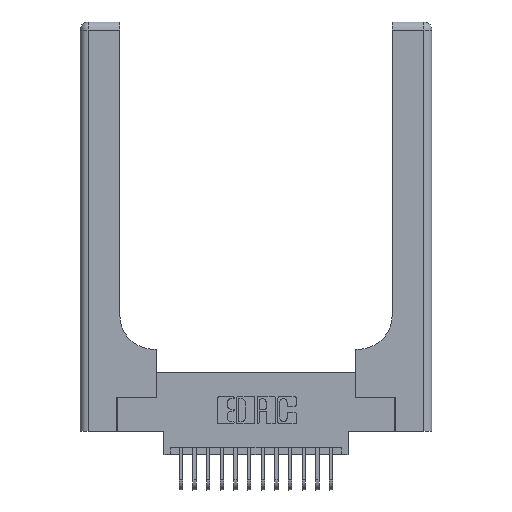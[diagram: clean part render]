
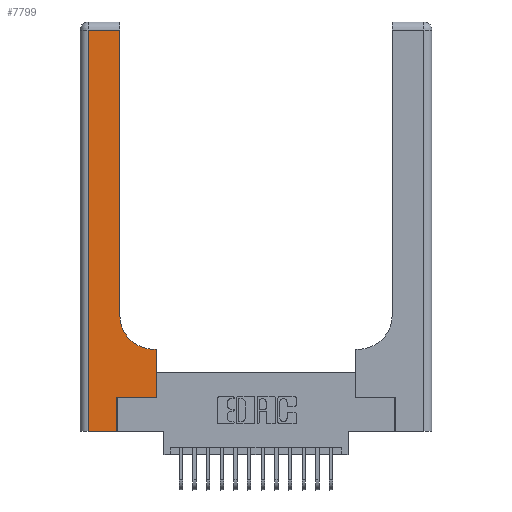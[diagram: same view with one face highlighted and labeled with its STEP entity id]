
A CAD part, top view. The second image highlights one B-rep face of the part: STEP entity #7799.
In plain terms, the highlighted planar face has unit normal (0, 0, 1).
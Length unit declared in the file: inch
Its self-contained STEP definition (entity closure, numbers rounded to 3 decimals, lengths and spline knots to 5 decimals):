
#319 = ORIENTED_EDGE ( 'NONE', *, *, #11639, .T. ) ;
#461 = CARTESIAN_POINT ( 'NONE',  ( 0.5415, 0.6, 0.37 ) ) ;
#698 = DIRECTION ( 'NONE',  ( 1., 0., 0. ) ) ;
#821 = LINE ( 'NONE', #3214, #14361 ) ;
#896 = CARTESIAN_POINT ( 'NONE',  ( 0.5585, 0.25, 0.37 ) ) ;
#969 = CARTESIAN_POINT ( 'NONE',  ( 0.5585, 0.6, 0.37 ) ) ;
#1005 = ORIENTED_EDGE ( 'NONE', *, *, #5511, .T. ) ;
#1983 = VECTOR ( 'NONE', #15180, 39.37008 ) ;
#2283 = VECTOR ( 'NONE', #18914, 39.37008 ) ;
#2351 = VERTEX_POINT ( 'NONE', #13773 ) ;
#3214 = CARTESIAN_POINT ( 'NONE',  ( 0.5585, 0.25, 0.37 ) ) ;
#3375 = CARTESIAN_POINT ( 'NONE',  ( 0., 2.94, 0.37 ) ) ;
#3940 = CARTESIAN_POINT ( 'NONE',  ( 0., 3., 0.37 ) ) ;
#4143 = CARTESIAN_POINT ( 'NONE',  ( 0.06, 0., 0.37 ) ) ;
#4503 = AXIS2_PLACEMENT_3D ( 'NONE', #3940, #8648, #5467 ) ;
#4760 = CARTESIAN_POINT ( 'NONE',  ( 0.06, 3., 0.37 ) ) ;
#4911 = EDGE_CURVE ( 'NONE', #13485, #12290, #10559, .T. ) ;
#5210 = VERTEX_POINT ( 'NONE', #969 ) ;
#5383 = ORIENTED_EDGE ( 'NONE', *, *, #13091, .T. ) ;
#5421 = EDGE_CURVE ( 'NONE', #14500, #8897, #20079, .T. ) ;
#5467 = DIRECTION ( 'NONE',  ( -1., 0., 0. ) ) ;
#5511 = EDGE_CURVE ( 'NONE', #2351, #17163, #15092, .T. ) ;
#5635 = VECTOR ( 'NONE', #9847, 39.37008 ) ;
#6227 = ORIENTED_EDGE ( 'NONE', *, *, #5421, .T. ) ;
#6395 = DIRECTION ( 'NONE',  ( 0., -1., 0. ) ) ;
#7012 = PLANE ( 'NONE',  #4503 ) ;
#7024 = ORIENTED_EDGE ( 'NONE', *, *, #4911, .T. ) ;
#7799 = ADVANCED_FACE ( 'NONE', ( #11246 ), #7012, .F. ) ;
#8013 = AXIS2_PLACEMENT_3D ( 'NONE', #13181, #8517, #698 ) ;
#8517 = DIRECTION ( 'NONE',  ( 0., 0., -1. ) ) ;
#8648 = DIRECTION ( 'NONE',  ( 0., 0., -1. ) ) ;
#8660 = DIRECTION ( 'NONE',  ( 0., 1., 0. ) ) ;
#8891 = CARTESIAN_POINT ( 'NONE',  ( 0.2915, 3., 0.37 ) ) ;
#8897 = VERTEX_POINT ( 'NONE', #4143 ) ;
#9036 = DIRECTION ( 'NONE',  ( 1., 0., 0. ) ) ;
#9175 = DIRECTION ( 'NONE',  ( -1., 0., 0. ) ) ;
#9626 = CARTESIAN_POINT ( 'NONE',  ( 0.269, 0.25, 0.37 ) ) ;
#9847 = DIRECTION ( 'NONE',  ( 0., 1., 0. ) ) ;
#10187 = CARTESIAN_POINT ( 'NONE',  ( 0.2915, 0.85, 0.37 ) ) ;
#10559 = CIRCLE ( 'NONE', #8013, 0.25 ) ;
#10997 = VECTOR ( 'NONE', #9036, 39.37008 ) ;
#11194 = VERTEX_POINT ( 'NONE', #15210 ) ;
#11246 = FACE_OUTER_BOUND ( 'NONE', #16853, .T. ) ;
#11639 = EDGE_CURVE ( 'NONE', #5210, #13485, #11757, .T. ) ;
#11698 = ORIENTED_EDGE ( 'NONE', *, *, #12469, .T. ) ;
#11757 = LINE ( 'NONE', #15244, #1983 ) ;
#11775 = ORIENTED_EDGE ( 'NONE', *, *, #16402, .T. ) ;
#12290 = VERTEX_POINT ( 'NONE', #10187 ) ;
#12469 = EDGE_CURVE ( 'NONE', #8897, #11194, #13225, .T. ) ;
#12474 = LINE ( 'NONE', #8891, #12969 ) ;
#12476 = CARTESIAN_POINT ( 'NONE',  ( 0.06, 2.94, 0.37 ) ) ;
#12969 = VECTOR ( 'NONE', #8660, 39.37008 ) ;
#13091 = EDGE_CURVE ( 'NONE', #11194, #2351, #19237, .T. ) ;
#13181 = CARTESIAN_POINT ( 'NONE',  ( 0.5415, 0.85, 0.37 ) ) ;
#13225 = LINE ( 'NONE', #18728, #10997 ) ;
#13485 = VERTEX_POINT ( 'NONE', #461 ) ;
#13773 = CARTESIAN_POINT ( 'NONE',  ( 0.269, 0.25, 0.37 ) ) ;
#13848 = VECTOR ( 'NONE', #6395, 39.37008 ) ;
#14361 = VECTOR ( 'NONE', #19212, 39.37008 ) ;
#14413 = CARTESIAN_POINT ( 'NONE',  ( 0.269, 0., 0.37 ) ) ;
#14500 = VERTEX_POINT ( 'NONE', #12476 ) ;
#15092 = LINE ( 'NONE', #9626, #2283 ) ;
#15125 = VECTOR ( 'NONE', #9175, 39.37008 ) ;
#15180 = DIRECTION ( 'NONE',  ( -1., 0., 0. ) ) ;
#15210 = CARTESIAN_POINT ( 'NONE',  ( 0.269, 0., 0.37 ) ) ;
#15244 = CARTESIAN_POINT ( 'NONE',  ( 0.2915, 0.6, 0.37 ) ) ;
#15332 = ORIENTED_EDGE ( 'NONE', *, *, #20327, .T. ) ;
#16402 = EDGE_CURVE ( 'NONE', #12290, #16723, #12474, .T. ) ;
#16723 = VERTEX_POINT ( 'NONE', #19732 ) ;
#16853 = EDGE_LOOP ( 'NONE', ( #11775, #19236, #6227, #11698, #5383, #1005, #15332, #319, #7024 ) ) ;
#17163 = VERTEX_POINT ( 'NONE', #896 ) ;
#18728 = CARTESIAN_POINT ( 'NONE',  ( 0., 0., 0.37 ) ) ;
#18914 = DIRECTION ( 'NONE',  ( 1., 0., 0. ) ) ;
#19212 = DIRECTION ( 'NONE',  ( 0., 1., 0. ) ) ;
#19236 = ORIENTED_EDGE ( 'NONE', *, *, #19681, .T. ) ;
#19237 = LINE ( 'NONE', #14413, #5635 ) ;
#19681 = EDGE_CURVE ( 'NONE', #16723, #14500, #19860, .T. ) ;
#19732 = CARTESIAN_POINT ( 'NONE',  ( 0.2915, 2.94, 0.37 ) ) ;
#19860 = LINE ( 'NONE', #3375, #15125 ) ;
#20079 = LINE ( 'NONE', #4760, #13848 ) ;
#20327 = EDGE_CURVE ( 'NONE', #17163, #5210, #821, .T. ) ;
